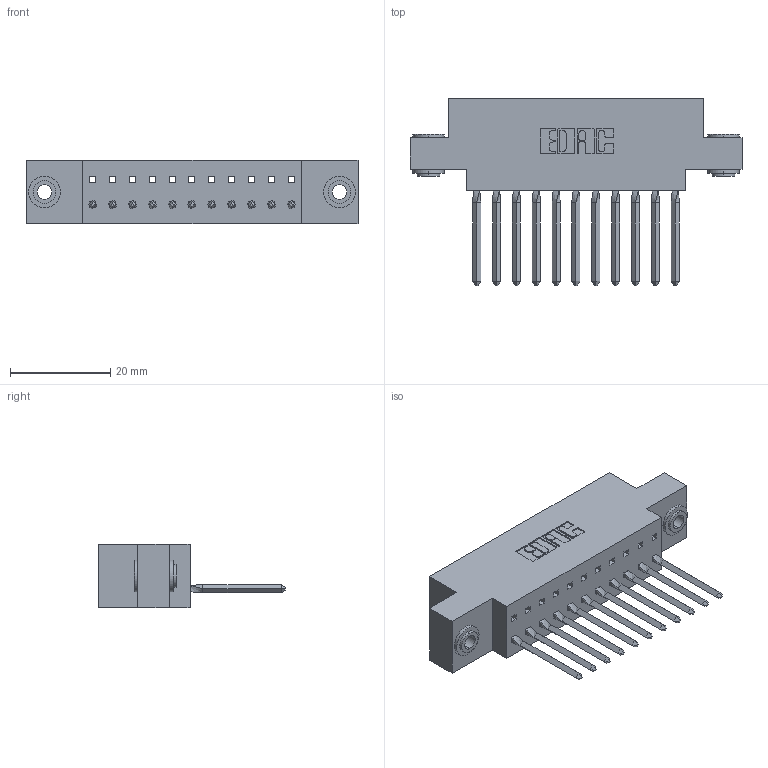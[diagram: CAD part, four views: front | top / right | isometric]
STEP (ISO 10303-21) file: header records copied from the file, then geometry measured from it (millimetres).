
FILE_DESCRIPTION (( 'STEP AP203' ), '1' );
FILE_NAME ('317-011-542-603.STEP', '2020-02-27T13:39:48', ( '' ), ( '' ), 'SwSTEP 2.0', 'SolidWorks 2016', '' );
FILE_SCHEMA (( 'CONFIG_CONTROL_DESIGN' ));
Length unit declared in the file: inch
Products named in the file (4): 317-011-542-603; 317-290-003_542; 345-250-002_345-250-002-102; 317 Part_.156 Dia - TH
Assembly tree (14 placements, depth 2):
  317-011-542-603
    317 Part_.156 Dia - TH
    317-290-003_542  x11
    345-250-002_345-250-002-102  x2
Bounding box: 66.29 x 37.34 x 12.7 mm (x, y, z)
Volume: 9435.8 mm3; surface area: 11037.2 mm2
Topology: 14 solids, 14 shells, 965 faces, 2738 edges, 1770 vertices
Faces by surface type: plane 772, cylinder 141, bspline 44, cone 8
Entity records: 19540 total; most frequent: CARTESIAN_POINT 3673, ORIENTED_EDGE 3340, DIRECTION 2882, EDGE_CURVE 1670, VECTOR 1476, LINE 1476, VERTEX_POINT 1106, AXIS2_PLACEMENT_3D 703
